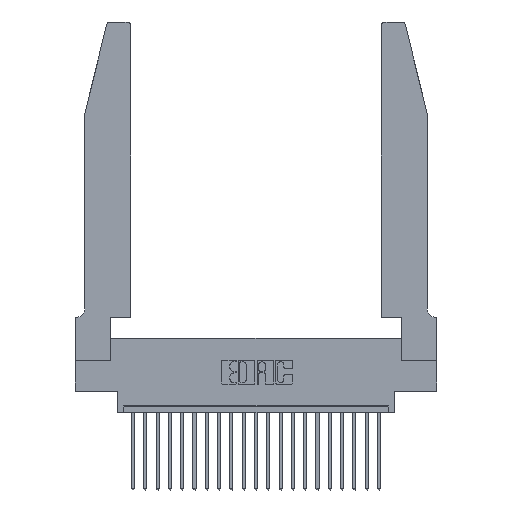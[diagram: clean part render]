
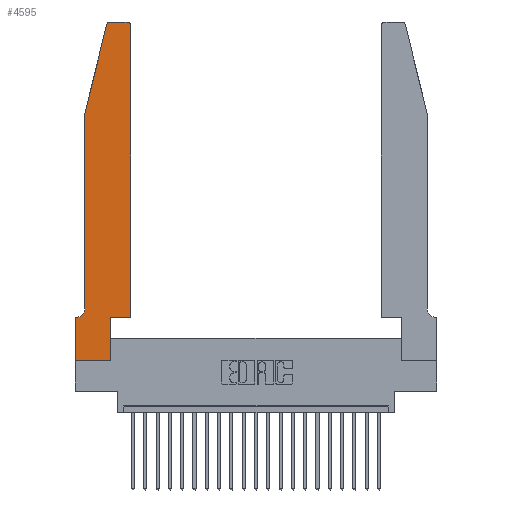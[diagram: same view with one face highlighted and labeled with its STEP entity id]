
A CAD part, top view. The second image highlights one B-rep face of the part: STEP entity #4595.
In plain terms, the highlighted planar face has unit normal (0, 0, 1).
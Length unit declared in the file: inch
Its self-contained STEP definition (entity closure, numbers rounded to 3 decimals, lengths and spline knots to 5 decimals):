
#338 = CARTESIAN_POINT ( 'NONE',  ( 0.0755, 0.42, 0.37 ) ) ;
#525 = VERTEX_POINT ( 'NONE', #3060 ) ;
#536 = EDGE_CURVE ( 'NONE', #7763, #5072, #9567, .T. ) ;
#594 = VERTEX_POINT ( 'NONE', #10838 ) ;
#1134 = EDGE_LOOP ( 'NONE', ( #17322, #5399, #3504, #6603, #15522, #21355, #17362, #23435, #13118, #4115, #21478, #15517 ) ) ;
#1650 = CARTESIAN_POINT ( 'NONE',  ( 0., 0., 0.37 ) ) ;
#2556 = VECTOR ( 'NONE', #4239, 39.37008 ) ;
#2782 = CARTESIAN_POINT ( 'NONE',  ( 0., 0., 0.37 ) ) ;
#3060 = CARTESIAN_POINT ( 'NONE',  ( 0.4505, 2.72, 0.37 ) ) ;
#3202 = AXIS2_PLACEMENT_3D ( 'NONE', #22113, #21870, #11066 ) ;
#3279 = AXIS2_PLACEMENT_3D ( 'NONE', #17531, #17458, #16059 ) ;
#3504 = ORIENTED_EDGE ( 'NONE', *, *, #5278, .T. ) ;
#3664 = VECTOR ( 'NONE', #22637, 39.37008 ) ;
#4009 = EDGE_CURVE ( 'NONE', #15544, #4733, #21378, .T. ) ;
#4011 = DIRECTION ( 'NONE',  ( -1., 0., 0. ) ) ;
#4115 = ORIENTED_EDGE ( 'NONE', *, *, #9437, .T. ) ;
#4239 = DIRECTION ( 'NONE',  ( 0., -1., 0. ) ) ;
#4595 = ADVANCED_FACE ( 'NONE', ( #5118 ), #4713, .T. ) ;
#4713 = PLANE ( 'NONE',  #18070 ) ;
#4733 = VERTEX_POINT ( 'NONE', #9194 ) ;
#5072 = VERTEX_POINT ( 'NONE', #7149 ) ;
#5091 = VERTEX_POINT ( 'NONE', #338 ) ;
#5118 = FACE_OUTER_BOUND ( 'NONE', #1134, .T. ) ;
#5132 = DIRECTION ( 'NONE',  ( 1., 0., 0. ) ) ;
#5275 = DIRECTION ( 'NONE',  ( 0., 1., 0. ) ) ;
#5278 = EDGE_CURVE ( 'NONE', #594, #11585, #19928, .T. ) ;
#5399 = ORIENTED_EDGE ( 'NONE', *, *, #16994, .T. ) ;
#5466 = EDGE_CURVE ( 'NONE', #6423, #20812, #13800, .T. ) ;
#6423 = VERTEX_POINT ( 'NONE', #6671 ) ;
#6603 = ORIENTED_EDGE ( 'NONE', *, *, #22717, .T. ) ;
#6671 = CARTESIAN_POINT ( 'NONE',  ( 0.2865, 0., 0.37 ) ) ;
#7149 = CARTESIAN_POINT ( 'NONE',  ( 0., 0.35, 0.37 ) ) ;
#7763 = VERTEX_POINT ( 'NONE', #12812 ) ;
#8179 = EDGE_CURVE ( 'NONE', #8800, #6423, #13552, .T. ) ;
#8379 = CARTESIAN_POINT ( 'NONE',  ( 0., 0.35, 0.37 ) ) ;
#8764 = CARTESIAN_POINT ( 'NONE',  ( 0.0755, 2., 0.37 ) ) ;
#8800 = VERTEX_POINT ( 'NONE', #2782 ) ;
#8838 = DIRECTION ( 'NONE',  ( -1., 0., 0. ) ) ;
#9001 = CARTESIAN_POINT ( 'NONE',  ( 0.2605, 2.75, 0.37 ) ) ;
#9194 = CARTESIAN_POINT ( 'NONE',  ( 0.284, 2.75, 0.37 ) ) ;
#9437 = EDGE_CURVE ( 'NONE', #20812, #18170, #14908, .T. ) ;
#9528 = CIRCLE ( 'NONE', #3279, 0.03 ) ;
#9567 = LINE ( 'NONE', #13109, #17547 ) ;
#10486 = DIRECTION ( 'NONE',  ( 0., 0., -1. ) ) ;
#10496 = EDGE_CURVE ( 'NONE', #18170, #525, #17381, .T. ) ;
#10701 = EDGE_CURVE ( 'NONE', #5072, #8800, #22182, .T. ) ;
#10838 = CARTESIAN_POINT ( 'NONE',  ( 0.25487, 2.72718, 0.37 ) ) ;
#11066 = DIRECTION ( 'NONE',  ( 1., 0., 0. ) ) ;
#11585 = VERTEX_POINT ( 'NONE', #20213 ) ;
#11742 = VECTOR ( 'NONE', #8838, 39.37008 ) ;
#11892 = EDGE_CURVE ( 'NONE', #525, #15544, #18207, .T. ) ;
#12021 = DIRECTION ( 'NONE',  ( 0., 1., 0. ) ) ;
#12142 = VECTOR ( 'NONE', #21343, 39.37008 ) ;
#12295 = DIRECTION ( 'NONE',  ( 1., 0., 0. ) ) ;
#12812 = CARTESIAN_POINT ( 'NONE',  ( 0.0055, 0.35, 0.37 ) ) ;
#13109 = CARTESIAN_POINT ( 'NONE',  ( 0.0755, 0.35, 0.37 ) ) ;
#13118 = ORIENTED_EDGE ( 'NONE', *, *, #5466, .T. ) ;
#13552 = LINE ( 'NONE', #1650, #20359 ) ;
#13713 = VECTOR ( 'NONE', #12021, 39.37008 ) ;
#13800 = LINE ( 'NONE', #19782, #20031 ) ;
#13895 = DIRECTION ( 'NONE',  ( 1., 0., 0. ) ) ;
#14095 = DIRECTION ( 'NONE',  ( -1., 0., 0. ) ) ;
#14908 = LINE ( 'NONE', #17369, #23382 ) ;
#15517 = ORIENTED_EDGE ( 'NONE', *, *, #11892, .T. ) ;
#15522 = ORIENTED_EDGE ( 'NONE', *, *, #22231, .T. ) ;
#15544 = VERTEX_POINT ( 'NONE', #19953 ) ;
#15638 = CARTESIAN_POINT ( 'NONE',  ( 0.4505, 0.35, 0.37 ) ) ;
#16059 = DIRECTION ( 'NONE',  ( 1., 0., 0. ) ) ;
#16994 = EDGE_CURVE ( 'NONE', #4733, #594, #9528, .T. ) ;
#17322 = ORIENTED_EDGE ( 'NONE', *, *, #4009, .T. ) ;
#17362 = ORIENTED_EDGE ( 'NONE', *, *, #10701, .T. ) ;
#17369 = CARTESIAN_POINT ( 'NONE',  ( 0.4505, 0.35, 0.37 ) ) ;
#17381 = LINE ( 'NONE', #15638, #13713 ) ;
#17458 = DIRECTION ( 'NONE',  ( 0., 0., 1. ) ) ;
#17531 = CARTESIAN_POINT ( 'NONE',  ( 0.284, 2.72, 0.37 ) ) ;
#17547 = VECTOR ( 'NONE', #4011, 39.37008 ) ;
#18070 = AXIS2_PLACEMENT_3D ( 'NONE', #8379, #21110, #12295 ) ;
#18170 = VERTEX_POINT ( 'NONE', #22294 ) ;
#18207 = CIRCLE ( 'NONE', #3202, 0.03 ) ;
#18800 = AXIS2_PLACEMENT_3D ( 'NONE', #21279, #10486, #14095 ) ;
#19073 = CARTESIAN_POINT ( 'NONE',  ( 0.2865, 0.35, 0.37 ) ) ;
#19782 = CARTESIAN_POINT ( 'NONE',  ( 0.2865, 0.35, 0.37 ) ) ;
#19928 = LINE ( 'NONE', #20755, #3664 ) ;
#19953 = CARTESIAN_POINT ( 'NONE',  ( 0.4205, 2.75, 0.37 ) ) ;
#20031 = VECTOR ( 'NONE', #5275, 39.37008 ) ;
#20112 = LINE ( 'NONE', #8764, #12142 ) ;
#20213 = CARTESIAN_POINT ( 'NONE',  ( 0.0755, 2., 0.37 ) ) ;
#20359 = VECTOR ( 'NONE', #5132, 39.37008 ) ;
#20715 = CARTESIAN_POINT ( 'NONE',  ( 0., 0., 0.37 ) ) ;
#20755 = CARTESIAN_POINT ( 'NONE',  ( 0.0755, 2., 0.37 ) ) ;
#20812 = VERTEX_POINT ( 'NONE', #19073 ) ;
#21110 = DIRECTION ( 'NONE',  ( 0., 0., 1. ) ) ;
#21279 = CARTESIAN_POINT ( 'NONE',  ( 0.0055, 0.42, 0.37 ) ) ;
#21343 = DIRECTION ( 'NONE',  ( 0., -1., 0. ) ) ;
#21355 = ORIENTED_EDGE ( 'NONE', *, *, #536, .T. ) ;
#21378 = LINE ( 'NONE', #9001, #11742 ) ;
#21478 = ORIENTED_EDGE ( 'NONE', *, *, #10496, .T. ) ;
#21870 = DIRECTION ( 'NONE',  ( 0., 0., 1. ) ) ;
#22113 = CARTESIAN_POINT ( 'NONE',  ( 0.4205, 2.72, 0.37 ) ) ;
#22182 = LINE ( 'NONE', #20715, #2556 ) ;
#22231 = EDGE_CURVE ( 'NONE', #5091, #7763, #22666, .T. ) ;
#22294 = CARTESIAN_POINT ( 'NONE',  ( 0.4505, 0.35, 0.37 ) ) ;
#22637 = DIRECTION ( 'NONE',  ( -0.239, -0.971, 0. ) ) ;
#22666 = CIRCLE ( 'NONE', #18800, 0.07 ) ;
#22717 = EDGE_CURVE ( 'NONE', #11585, #5091, #20112, .T. ) ;
#23382 = VECTOR ( 'NONE', #13895, 39.37008 ) ;
#23435 = ORIENTED_EDGE ( 'NONE', *, *, #8179, .T. ) ;
